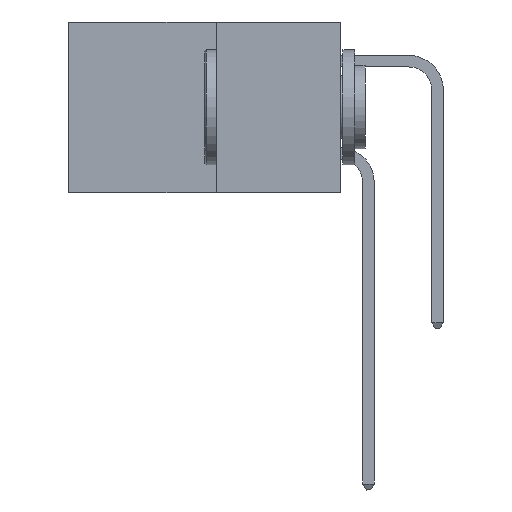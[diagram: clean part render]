
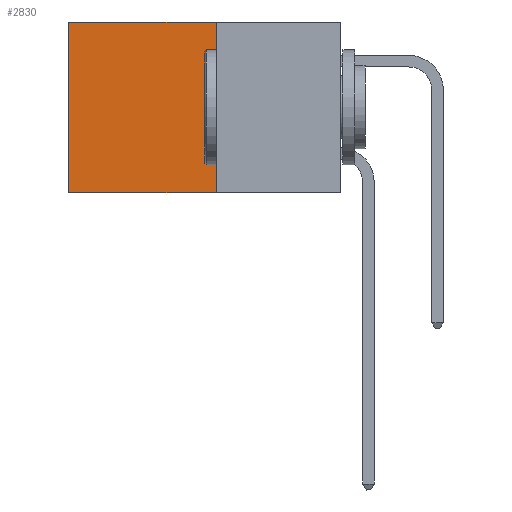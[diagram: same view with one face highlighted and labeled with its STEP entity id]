
A CAD part, left-side view. The second image highlights one B-rep face of the part: STEP entity #2830.
In plain terms, the highlighted planar face has unit normal (-1, 0, 0).
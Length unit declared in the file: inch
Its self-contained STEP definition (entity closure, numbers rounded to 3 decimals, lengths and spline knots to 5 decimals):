
#32 = VECTOR ( 'NONE', #2587, 39.37008 ) ;
#1006 = ORIENTED_EDGE ( 'NONE', *, *, #1415, .F. ) ;
#1098 = ORIENTED_EDGE ( 'NONE', *, *, #7737, .F. ) ;
#1273 = FACE_OUTER_BOUND ( 'NONE', #11002, .T. ) ;
#1304 = VECTOR ( 'NONE', #5139, 39.37008 ) ;
#1372 = ORIENTED_EDGE ( 'NONE', *, *, #5344, .T. ) ;
#1415 = EDGE_CURVE ( 'NONE', #6369, #7858, #6513, .T. ) ;
#1683 = DIRECTION ( 'NONE',  ( 0., 1., 0. ) ) ;
#1692 = CARTESIAN_POINT ( 'NONE',  ( 0.277, 0.27, -0.37 ) ) ;
#1802 = VECTOR ( 'NONE', #7802, 39.37008 ) ;
#2237 = CARTESIAN_POINT ( 'NONE',  ( 0.277, 0.59, -0.37 ) ) ;
#2387 = CARTESIAN_POINT ( 'NONE',  ( 0.277, 0.27, -0.37 ) ) ;
#2517 = LINE ( 'NONE', #2738, #32 ) ;
#2521 = VERTEX_POINT ( 'NONE', #7524 ) ;
#2556 = VERTEX_POINT ( 'NONE', #2237 ) ;
#2587 = DIRECTION ( 'NONE',  ( 0., 1., 0. ) ) ;
#2738 = CARTESIAN_POINT ( 'NONE',  ( 0.277, 0.27, 0. ) ) ;
#2830 = ADVANCED_FACE ( 'NONE', ( #1273 ), #4566, .F. ) ;
#3571 = DIRECTION ( 'NONE',  ( 1., 0., 0. ) ) ;
#3728 = VECTOR ( 'NONE', #1683, 39.37008 ) ;
#4566 = PLANE ( 'NONE',  #6342 ) ;
#5046 = CARTESIAN_POINT ( 'NONE',  ( 0.277, 0.27, -0.37 ) ) ;
#5139 = DIRECTION ( 'NONE',  ( 0., 0., -1. ) ) ;
#5344 = EDGE_CURVE ( 'NONE', #2521, #2556, #11448, .T. ) ;
#6342 = AXIS2_PLACEMENT_3D ( 'NONE', #1692, #3571, #10795 ) ;
#6369 = VERTEX_POINT ( 'NONE', #6501 ) ;
#6501 = CARTESIAN_POINT ( 'NONE',  ( 0.277, 0.27, 0. ) ) ;
#6513 = LINE ( 'NONE', #5046, #1304 ) ;
#6853 = EDGE_CURVE ( 'NONE', #6369, #2521, #2517, .T. ) ;
#7374 = ORIENTED_EDGE ( 'NONE', *, *, #6853, .T. ) ;
#7524 = CARTESIAN_POINT ( 'NONE',  ( 0.277, 0.59, 0. ) ) ;
#7737 = EDGE_CURVE ( 'NONE', #7858, #2556, #10893, .T. ) ;
#7802 = DIRECTION ( 'NONE',  ( 0., 0., -1. ) ) ;
#7858 = VERTEX_POINT ( 'NONE', #9429 ) ;
#7915 = CARTESIAN_POINT ( 'NONE',  ( 0.277, 0.59, -0.37 ) ) ;
#9429 = CARTESIAN_POINT ( 'NONE',  ( 0.277, 0.27, -0.37 ) ) ;
#10795 = DIRECTION ( 'NONE',  ( 0., 0., -1. ) ) ;
#10893 = LINE ( 'NONE', #2387, #3728 ) ;
#11002 = EDGE_LOOP ( 'NONE', ( #1372, #1098, #1006, #7374 ) ) ;
#11448 = LINE ( 'NONE', #7915, #1802 ) ;
